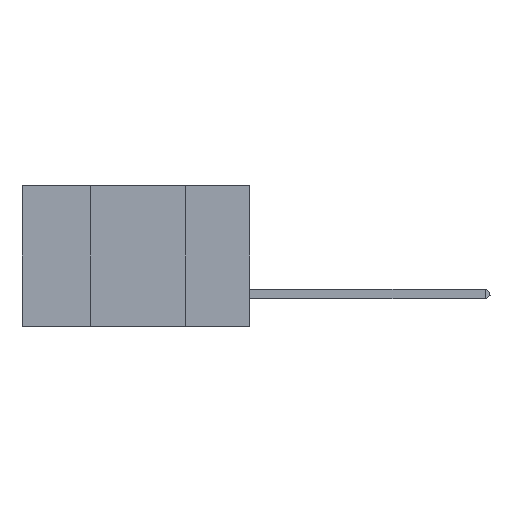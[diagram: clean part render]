
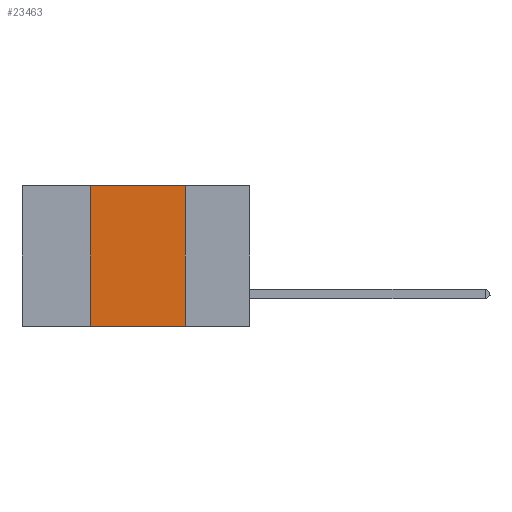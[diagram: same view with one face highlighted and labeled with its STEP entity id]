
A CAD part, left-side view. The second image highlights one B-rep face of the part: STEP entity #23463.
In plain terms, the highlighted planar face has unit normal (-1, 0, 0).
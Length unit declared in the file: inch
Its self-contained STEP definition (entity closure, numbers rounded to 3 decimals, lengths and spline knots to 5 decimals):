
#181 = VECTOR ( 'NONE', #11490, 39.37008 ) ;
#1855 = VECTOR ( 'NONE', #17443, 39.37008 ) ;
#2324 = VECTOR ( 'NONE', #24731, 39.37008 ) ;
#2872 = VERTEX_POINT ( 'NONE', #21356 ) ;
#3466 = CARTESIAN_POINT ( 'NONE',  ( 0., 0.6, 0. ) ) ;
#4491 = VERTEX_POINT ( 'NONE', #14879 ) ;
#4675 = ORIENTED_EDGE ( 'NONE', *, *, #14937, .F. ) ;
#5472 = EDGE_CURVE ( 'NONE', #12504, #8227, #21116, .T. ) ;
#5480 = ORIENTED_EDGE ( 'NONE', *, *, #5472, .F. ) ;
#7382 = LINE ( 'NONE', #20299, #2324 ) ;
#7654 = CARTESIAN_POINT ( 'NONE',  ( 0., 0.42, -0.37 ) ) ;
#7872 = LINE ( 'NONE', #9118, #1855 ) ;
#8227 = VERTEX_POINT ( 'NONE', #10045 ) ;
#9118 = CARTESIAN_POINT ( 'NONE',  ( 0., 0.17, 0. ) ) ;
#9406 = DIRECTION ( 'NONE',  ( 0., 0., -1. ) ) ;
#10045 = CARTESIAN_POINT ( 'NONE',  ( 0., 0.42, 0. ) ) ;
#10861 = DIRECTION ( 'NONE',  ( 0., 0., 1. ) ) ;
#11349 = DIRECTION ( 'NONE',  ( 1., 0., 0. ) ) ;
#11402 = AXIS2_PLACEMENT_3D ( 'NONE', #17457, #11349, #9406 ) ;
#11490 = DIRECTION ( 'NONE',  ( 0., -1., 0. ) ) ;
#12504 = VERTEX_POINT ( 'NONE', #7654 ) ;
#14879 = CARTESIAN_POINT ( 'NONE',  ( 0., 0.17, -0.37 ) ) ;
#14937 = EDGE_CURVE ( 'NONE', #2872, #4491, #7872, .T. ) ;
#15693 = LINE ( 'NONE', #3466, #181 ) ;
#16415 = EDGE_LOOP ( 'NONE', ( #4675, #25584, #5480, #22489 ) ) ;
#17443 = DIRECTION ( 'NONE',  ( 0., 0., -1. ) ) ;
#17457 = CARTESIAN_POINT ( 'NONE',  ( 0., 0.6, 0. ) ) ;
#18240 = VECTOR ( 'NONE', #10861, 39.37008 ) ;
#19099 = EDGE_CURVE ( 'NONE', #12504, #4491, #7382, .T. ) ;
#20299 = CARTESIAN_POINT ( 'NONE',  ( 0., 0.6, -0.37 ) ) ;
#20789 = CARTESIAN_POINT ( 'NONE',  ( 0., 0.42, 0. ) ) ;
#21116 = LINE ( 'NONE', #20789, #18240 ) ;
#21356 = CARTESIAN_POINT ( 'NONE',  ( 0., 0.17, 0. ) ) ;
#22489 = ORIENTED_EDGE ( 'NONE', *, *, #19099, .T. ) ;
#23463 = ADVANCED_FACE ( 'NONE', ( #26184 ), #25354, .F. ) ;
#24071 = EDGE_CURVE ( 'NONE', #8227, #2872, #15693, .T. ) ;
#24731 = DIRECTION ( 'NONE',  ( 0., -1., 0. ) ) ;
#25354 = PLANE ( 'NONE',  #11402 ) ;
#25584 = ORIENTED_EDGE ( 'NONE', *, *, #24071, .F. ) ;
#26184 = FACE_OUTER_BOUND ( 'NONE', #16415, .T. ) ;
